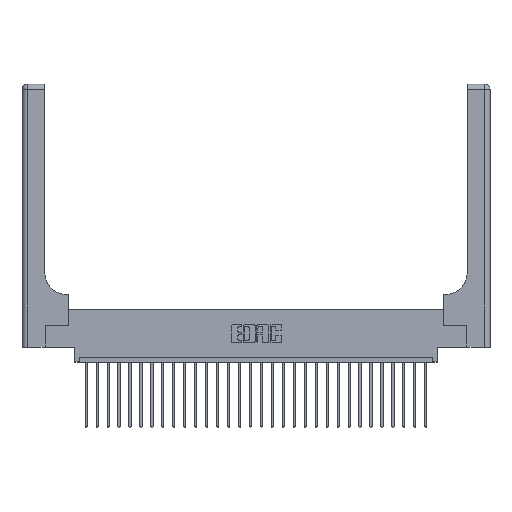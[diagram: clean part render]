
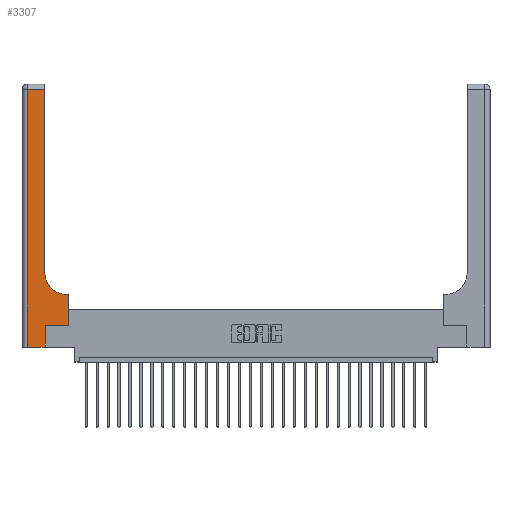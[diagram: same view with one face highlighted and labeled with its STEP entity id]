
A CAD part, top view. The second image highlights one B-rep face of the part: STEP entity #3307.
In plain terms, the highlighted planar face has unit normal (0, 0, 1).
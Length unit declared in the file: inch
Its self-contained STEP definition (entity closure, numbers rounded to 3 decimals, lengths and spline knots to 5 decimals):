
#590 = VERTEX_POINT ( 'NONE', #13351 ) ;
#1742 = CARTESIAN_POINT ( 'NONE',  ( 0.26, 0.6, 0.37 ) ) ;
#2186 = AXIS2_PLACEMENT_3D ( 'NONE', #12330, #20380, #10014 ) ;
#2250 = DIRECTION ( 'NONE',  ( 0., 0., -1. ) ) ;
#2337 = CARTESIAN_POINT ( 'NONE',  ( 0., 0., 0.37 ) ) ;
#3307 = ADVANCED_FACE ( 'NONE', ( #8807 ), #17112, .F. ) ;
#3348 = CARTESIAN_POINT ( 'NONE',  ( 0.265, 0.25, 0.37 ) ) ;
#3734 = VECTOR ( 'NONE', #13128, 39.37008 ) ;
#3740 = LINE ( 'NONE', #10134, #16771 ) ;
#4212 = ORIENTED_EDGE ( 'NONE', *, *, #15140, .T. ) ;
#4258 = CARTESIAN_POINT ( 'NONE',  ( 0.528, 0.25, 0.37 ) ) ;
#4286 = ORIENTED_EDGE ( 'NONE', *, *, #15721, .T. ) ;
#4550 = VECTOR ( 'NONE', #24531, 39.37008 ) ;
#4552 = ORIENTED_EDGE ( 'NONE', *, *, #7830, .T. ) ;
#5065 = VERTEX_POINT ( 'NONE', #24337 ) ;
#5099 = VECTOR ( 'NONE', #18795, 39.37008 ) ;
#5767 = VECTOR ( 'NONE', #17426, 39.37008 ) ;
#5960 = DIRECTION ( 'NONE',  ( -1., 0., 0. ) ) ;
#6131 = LINE ( 'NONE', #14313, #5099 ) ;
#6375 = VERTEX_POINT ( 'NONE', #4258 ) ;
#7653 = ORIENTED_EDGE ( 'NONE', *, *, #7936, .T. ) ;
#7830 = EDGE_CURVE ( 'NONE', #6375, #590, #12543, .T. ) ;
#7936 = EDGE_CURVE ( 'NONE', #9874, #9300, #6131, .T. ) ;
#8197 = VERTEX_POINT ( 'NONE', #9634 ) ;
#8368 = ORIENTED_EDGE ( 'NONE', *, *, #13656, .T. ) ;
#8807 = FACE_OUTER_BOUND ( 'NONE', #23856, .T. ) ;
#8849 = ORIENTED_EDGE ( 'NONE', *, *, #12110, .T. ) ;
#8937 = VECTOR ( 'NONE', #26517, 39.37008 ) ;
#8987 = CARTESIAN_POINT ( 'NONE',  ( 0.26, 3., 0.37 ) ) ;
#9300 = VERTEX_POINT ( 'NONE', #18218 ) ;
#9634 = CARTESIAN_POINT ( 'NONE',  ( 0.51, 0.6, 0.37 ) ) ;
#9874 = VERTEX_POINT ( 'NONE', #10268 ) ;
#10014 = DIRECTION ( 'NONE',  ( 1., 0., 0. ) ) ;
#10134 = CARTESIAN_POINT ( 'NONE',  ( 0.265, 0., 0.37 ) ) ;
#10268 = CARTESIAN_POINT ( 'NONE',  ( 0.06, 2.94, 0.37 ) ) ;
#10269 = LINE ( 'NONE', #12190, #8937 ) ;
#11219 = EDGE_CURVE ( 'NONE', #9300, #24335, #21036, .T. ) ;
#11922 = DIRECTION ( 'NONE',  ( 0., 1., 0. ) ) ;
#12110 = EDGE_CURVE ( 'NONE', #25587, #9874, #26169, .T. ) ;
#12190 = CARTESIAN_POINT ( 'NONE',  ( 0.265, 0.25, 0.37 ) ) ;
#12330 = CARTESIAN_POINT ( 'NONE',  ( 0.51, 0.85, 0.37 ) ) ;
#12543 = LINE ( 'NONE', #14438, #25567 ) ;
#12646 = CIRCLE ( 'NONE', #2186, 0.25 ) ;
#13128 = DIRECTION ( 'NONE',  ( 1., 0., 0. ) ) ;
#13351 = CARTESIAN_POINT ( 'NONE',  ( 0.528, 0.6, 0.37 ) ) ;
#13656 = EDGE_CURVE ( 'NONE', #5065, #25587, #23043, .T. ) ;
#14190 = VECTOR ( 'NONE', #5960, 39.37008 ) ;
#14313 = CARTESIAN_POINT ( 'NONE',  ( 0.06, 3., 0.37 ) ) ;
#14438 = CARTESIAN_POINT ( 'NONE',  ( 0.528, 0.25, 0.37 ) ) ;
#14535 = LINE ( 'NONE', #1742, #4550 ) ;
#15140 = EDGE_CURVE ( 'NONE', #590, #8197, #14535, .T. ) ;
#15388 = AXIS2_PLACEMENT_3D ( 'NONE', #25312, #2250, #25451 ) ;
#15713 = EDGE_CURVE ( 'NONE', #24335, #17051, #3740, .T. ) ;
#15721 = EDGE_CURVE ( 'NONE', #17051, #6375, #10269, .T. ) ;
#15762 = ORIENTED_EDGE ( 'NONE', *, *, #11219, .T. ) ;
#16186 = CARTESIAN_POINT ( 'NONE',  ( 0., 2.94, 0.37 ) ) ;
#16631 = ORIENTED_EDGE ( 'NONE', *, *, #18553, .T. ) ;
#16771 = VECTOR ( 'NONE', #11922, 39.37008 ) ;
#17051 = VERTEX_POINT ( 'NONE', #3348 ) ;
#17112 = PLANE ( 'NONE',  #15388 ) ;
#17426 = DIRECTION ( 'NONE',  ( 0., 1., 0. ) ) ;
#18218 = CARTESIAN_POINT ( 'NONE',  ( 0.06, 0., 0.37 ) ) ;
#18553 = EDGE_CURVE ( 'NONE', #8197, #5065, #12646, .T. ) ;
#18795 = DIRECTION ( 'NONE',  ( 0., -1., 0. ) ) ;
#20380 = DIRECTION ( 'NONE',  ( 0., 0., -1. ) ) ;
#20603 = CARTESIAN_POINT ( 'NONE',  ( 0.26, 2.94, 0.37 ) ) ;
#21036 = LINE ( 'NONE', #2337, #3734 ) ;
#22104 = CARTESIAN_POINT ( 'NONE',  ( 0.265, 0., 0.37 ) ) ;
#23043 = LINE ( 'NONE', #8987, #5767 ) ;
#23564 = ORIENTED_EDGE ( 'NONE', *, *, #15713, .T. ) ;
#23856 = EDGE_LOOP ( 'NONE', ( #8368, #8849, #7653, #15762, #23564, #4286, #4552, #4212, #16631 ) ) ;
#24335 = VERTEX_POINT ( 'NONE', #22104 ) ;
#24337 = CARTESIAN_POINT ( 'NONE',  ( 0.26, 0.85, 0.37 ) ) ;
#24531 = DIRECTION ( 'NONE',  ( -1., 0., 0. ) ) ;
#25312 = CARTESIAN_POINT ( 'NONE',  ( 0., 3., 0.37 ) ) ;
#25451 = DIRECTION ( 'NONE',  ( -1., 0., 0. ) ) ;
#25567 = VECTOR ( 'NONE', #26740, 39.37008 ) ;
#25587 = VERTEX_POINT ( 'NONE', #20603 ) ;
#26169 = LINE ( 'NONE', #16186, #14190 ) ;
#26517 = DIRECTION ( 'NONE',  ( 1., 0., 0. ) ) ;
#26740 = DIRECTION ( 'NONE',  ( 0., 1., 0. ) ) ;
